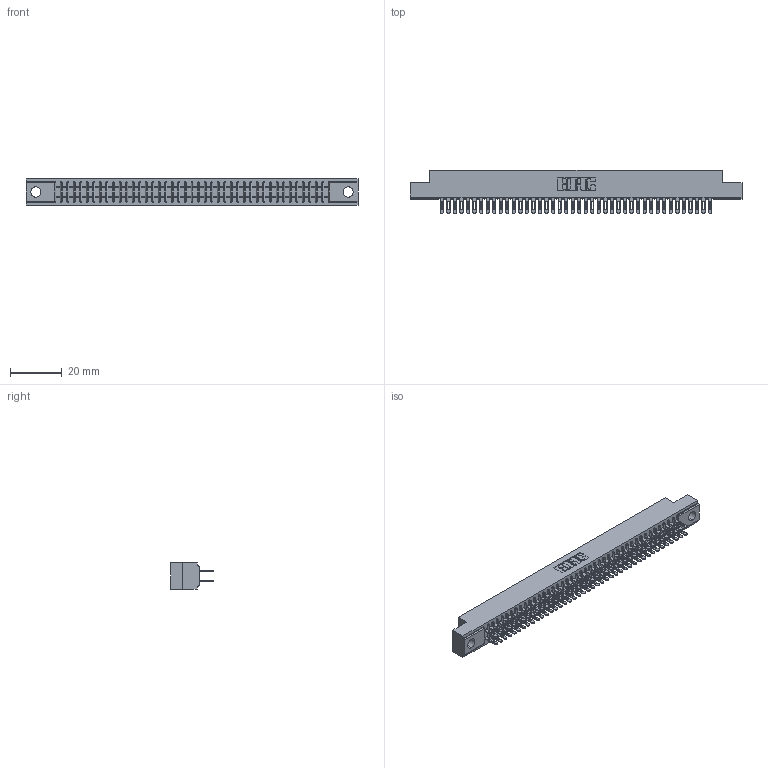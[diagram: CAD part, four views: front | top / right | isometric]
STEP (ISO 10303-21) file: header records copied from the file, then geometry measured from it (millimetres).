
FILE_DESCRIPTION (( 'STEP AP203' ), '1' );
FILE_NAME ('341-084-500-204.STEP', '2018-08-07T22:27:43', ( '' ), ( '' ), 'SwSTEP 2.0', 'SolidWorks 2016', '' );
FILE_SCHEMA (( 'CONFIG_CONTROL_DESIGN' ));
Length unit declared in the file: inch
Products named in the file (3): 341 Part_.156 (3.96) Dia Mounting Holes; 341-292-001_341-292-100; 341-084-500-204
Assembly tree (85 placements, depth 2):
  341-084-500-204
    341 Part_.156 (3.96) Dia Mounting Holes
    341-292-001_341-292-100  x84
Bounding box: 128.91 x 16.69 x 10.16 mm (x, y, z)
Volume: 9521.5 mm3; surface area: 17488.7 mm2
Topology: 85 solids, 85 shells, 5674 faces, 16438 edges, 10646 vertices
Faces by surface type: plane 3274, cylinder 2232, sphere 86, torus 82
Entity records: 51255 total; most frequent: CARTESIAN_POINT 8524, ORIENTED_EDGE 8468, DIRECTION 8268, EDGE_CURVE 4234, LINE 3424, VECTOR 3424, VERTEX_POINT 2678, AXIS2_PLACEMENT_3D 2422
